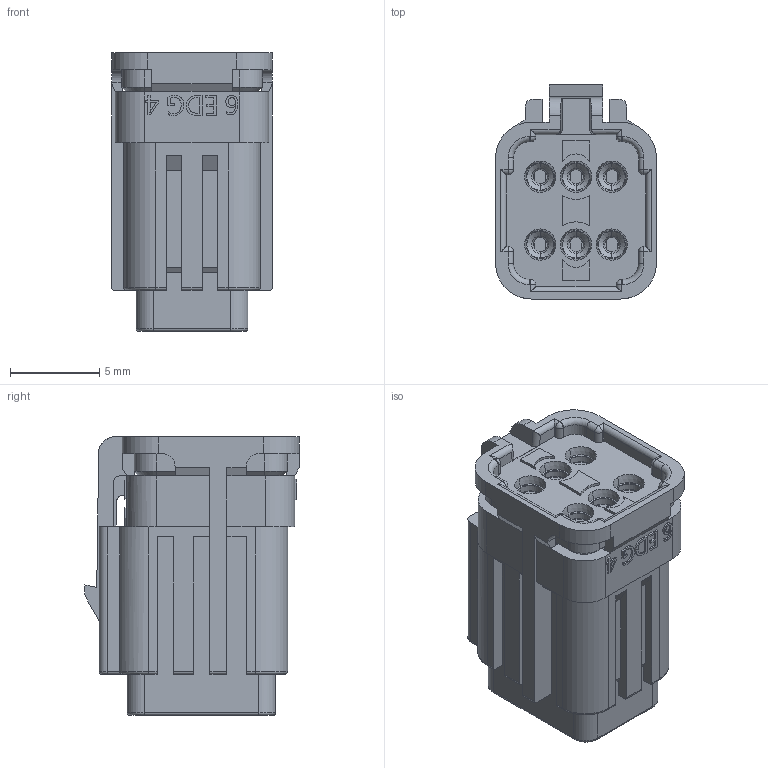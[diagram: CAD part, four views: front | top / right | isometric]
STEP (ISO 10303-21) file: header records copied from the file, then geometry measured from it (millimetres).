
FILE_DESCRIPTION (( 'STEP AP203' ), '1' );
FILE_NAME ('566-006-000-810.STEP', '2021-10-08T14:53:03', ( '' ), ( '' ), 'SwSTEP 2.0', 'SolidWorks 2020', '' );
FILE_SCHEMA (( 'CONFIG_CONTROL_DESIGN' ));
Length unit declared in the file: millimetre
Products named in the file (1): 566-006-000-810
Bounding box: 9 x 12 x 15.6 mm (x, y, z)
Volume: 953.6 mm3; surface area: 1588.7 mm2
Topology: 2 solids, 8 shells, 1147 faces, 2898 edges, 1778 vertices
Faces by surface type: plane 689, torus 182, cylinder 164, cone 64, bspline 40, sphere 8
Entity records: 35945 total; most frequent: CARTESIAN_POINT 8252, ORIENTED_EDGE 5780, DIRECTION 5714, EDGE_CURVE 2890, LINE 2082, VECTOR 2082, AXIS2_PLACEMENT_3D 1816, VERTEX_POINT 1778
